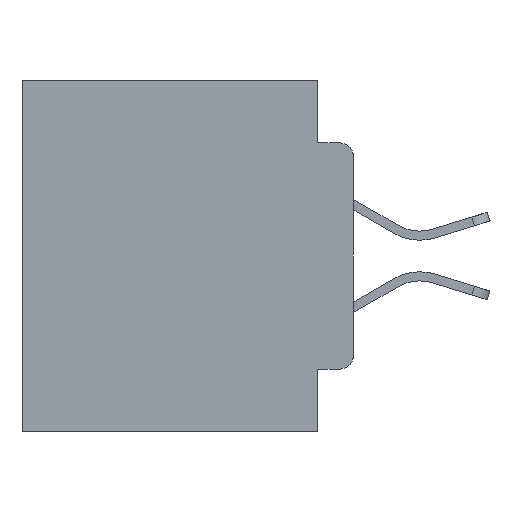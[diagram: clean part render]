
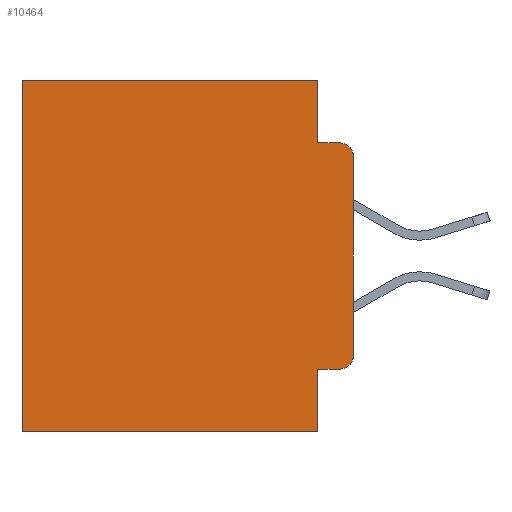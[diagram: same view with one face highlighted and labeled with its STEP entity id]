
A CAD part, left-side view. The second image highlights one B-rep face of the part: STEP entity #10464.
In plain terms, the highlighted planar face has unit normal (-1, 0, 0).
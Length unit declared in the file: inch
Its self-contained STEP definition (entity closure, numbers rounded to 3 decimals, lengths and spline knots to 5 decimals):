
#83 = EDGE_CURVE ( 'NONE', #1713, #8962, #18063, .T. ) ;
#422 = CARTESIAN_POINT ( 'NONE',  ( 0.298, 0.473, -0.5 ) ) ;
#614 = ORIENTED_EDGE ( 'NONE', *, *, #17056, .T. ) ;
#1175 = DIRECTION ( 'NONE',  ( 0., -1., 0. ) ) ;
#1609 = EDGE_CURVE ( 'NONE', #19497, #1713, #21228, .T. ) ;
#1713 = VERTEX_POINT ( 'NONE', #23904 ) ;
#1813 = ORIENTED_EDGE ( 'NONE', *, *, #6342, .T. ) ;
#1899 = ORIENTED_EDGE ( 'NONE', *, *, #4800, .F. ) ;
#2069 = VERTEX_POINT ( 'NONE', #6757 ) ;
#2101 = CARTESIAN_POINT ( 'NONE',  ( 0.298, 0.473, 0. ) ) ;
#2574 = DIRECTION ( 'NONE',  ( -1., 0., 0. ) ) ;
#2893 = VECTOR ( 'NONE', #25058, 39.37008 ) ;
#3018 = EDGE_CURVE ( 'NONE', #2069, #7826, #5050, .T. ) ;
#3116 = DIRECTION ( 'NONE',  ( 0., 1., 0. ) ) ;
#3184 = ORIENTED_EDGE ( 'NONE', *, *, #10996, .F. ) ;
#3224 = CARTESIAN_POINT ( 'NONE',  ( 0.298, 0., 0. ) ) ;
#3496 = VECTOR ( 'NONE', #6843, 39.37008 ) ;
#3650 = EDGE_LOOP ( 'NONE', ( #3685, #614, #3184, #29299, #12948, #1813, #5526, #1899, #18393, #23657 ) ) ;
#3685 = ORIENTED_EDGE ( 'NONE', *, *, #24671, .F. ) ;
#4800 = EDGE_CURVE ( 'NONE', #19497, #2069, #6781, .T. ) ;
#5050 = LINE ( 'NONE', #26342, #21846 ) ;
#5526 = ORIENTED_EDGE ( 'NONE', *, *, #3018, .F. ) ;
#5984 = EDGE_CURVE ( 'NONE', #28647, #21015, #12201, .T. ) ;
#6342 = EDGE_CURVE ( 'NONE', #21015, #7826, #27037, .T. ) ;
#6757 = CARTESIAN_POINT ( 'NONE',  ( 0.298, 0.051, -0.5 ) ) ;
#6781 = LINE ( 'NONE', #16631, #23544 ) ;
#6843 = DIRECTION ( 'NONE',  ( 0., 0., -1. ) ) ;
#7109 = DIRECTION ( 'NONE',  ( 0., 0., -1. ) ) ;
#7826 = VERTEX_POINT ( 'NONE', #422 ) ;
#8467 = CARTESIAN_POINT ( 'NONE',  ( 0.298, 0.051, -0.4115 ) ) ;
#8962 = VERTEX_POINT ( 'NONE', #25140 ) ;
#9203 = VERTEX_POINT ( 'NONE', #17669 ) ;
#9458 = EDGE_CURVE ( 'NONE', #28647, #9203, #14179, .T. ) ;
#9482 = CARTESIAN_POINT ( 'NONE',  ( 0.298, 0., -0.1085 ) ) ;
#9859 = AXIS2_PLACEMENT_3D ( 'NONE', #20017, #26807, #13266 ) ;
#10336 = CARTESIAN_POINT ( 'NONE',  ( 0.298, 0.02, -0.3915 ) ) ;
#10464 = ADVANCED_FACE ( 'NONE', ( #17997 ), #10997, .F. ) ;
#10515 = LINE ( 'NONE', #12737, #15847 ) ;
#10679 = VERTEX_POINT ( 'NONE', #9482 ) ;
#10996 = EDGE_CURVE ( 'NONE', #9203, #28455, #10515, .T. ) ;
#10997 = PLANE ( 'NONE',  #9859 ) ;
#11838 = CARTESIAN_POINT ( 'NONE',  ( 0.298, 0., 0. ) ) ;
#12201 = LINE ( 'NONE', #11838, #24267 ) ;
#12324 = CARTESIAN_POINT ( 'NONE',  ( 0.298, 0.02, -0.1085 ) ) ;
#12666 = CARTESIAN_POINT ( 'NONE',  ( 0.298, 0.051, 0. ) ) ;
#12737 = CARTESIAN_POINT ( 'NONE',  ( 0.298, 0.051, -0.0885 ) ) ;
#12948 = ORIENTED_EDGE ( 'NONE', *, *, #5984, .T. ) ;
#13078 = DIRECTION ( 'NONE',  ( 0., 0., -1. ) ) ;
#13266 = DIRECTION ( 'NONE',  ( 0., 0., -1. ) ) ;
#14179 = LINE ( 'NONE', #23072, #26190 ) ;
#14617 = DIRECTION ( 'NONE',  ( 0., 0., -1. ) ) ;
#14702 = DIRECTION ( 'NONE',  ( 0., 1., 0. ) ) ;
#15847 = VECTOR ( 'NONE', #1175, 39.37008 ) ;
#16631 = CARTESIAN_POINT ( 'NONE',  ( 0.298, 0.051, 0. ) ) ;
#17056 = EDGE_CURVE ( 'NONE', #10679, #28455, #18726, .T. ) ;
#17188 = DIRECTION ( 'NONE',  ( 0., 0., -1. ) ) ;
#17296 = CARTESIAN_POINT ( 'NONE',  ( 0.298, 0.473, 0. ) ) ;
#17669 = CARTESIAN_POINT ( 'NONE',  ( 0.298, 0.051, -0.0885 ) ) ;
#17997 = FACE_OUTER_BOUND ( 'NONE', #3650, .T. ) ;
#18063 = CIRCLE ( 'NONE', #24519, 0.02 ) ;
#18393 = ORIENTED_EDGE ( 'NONE', *, *, #1609, .T. ) ;
#18726 = CIRCLE ( 'NONE', #27370, 0.02 ) ;
#18839 = CARTESIAN_POINT ( 'NONE',  ( 0.298, 0.02, -0.0885 ) ) ;
#19280 = DIRECTION ( 'NONE',  ( 0., 0., -1. ) ) ;
#19497 = VERTEX_POINT ( 'NONE', #22235 ) ;
#20017 = CARTESIAN_POINT ( 'NONE',  ( 0.298, 0., 0. ) ) ;
#21015 = VERTEX_POINT ( 'NONE', #17296 ) ;
#21228 = LINE ( 'NONE', #8467, #2893 ) ;
#21846 = VECTOR ( 'NONE', #3116, 39.37008 ) ;
#22235 = CARTESIAN_POINT ( 'NONE',  ( 0.298, 0.051, -0.4115 ) ) ;
#23072 = CARTESIAN_POINT ( 'NONE',  ( 0.298, 0.051, 0. ) ) ;
#23544 = VECTOR ( 'NONE', #17188, 39.37008 ) ;
#23657 = ORIENTED_EDGE ( 'NONE', *, *, #83, .T. ) ;
#23904 = CARTESIAN_POINT ( 'NONE',  ( 0.298, 0.02, -0.4115 ) ) ;
#24267 = VECTOR ( 'NONE', #14702, 39.37008 ) ;
#24389 = VECTOR ( 'NONE', #19280, 39.37008 ) ;
#24519 = AXIS2_PLACEMENT_3D ( 'NONE', #10336, #2574, #13078 ) ;
#24671 = EDGE_CURVE ( 'NONE', #10679, #8962, #25117, .T. ) ;
#25058 = DIRECTION ( 'NONE',  ( 0., -1., 0. ) ) ;
#25117 = LINE ( 'NONE', #3224, #24389 ) ;
#25140 = CARTESIAN_POINT ( 'NONE',  ( 0.298, 0., -0.3915 ) ) ;
#26190 = VECTOR ( 'NONE', #7109, 39.37008 ) ;
#26342 = CARTESIAN_POINT ( 'NONE',  ( 0.298, 0., -0.5 ) ) ;
#26807 = DIRECTION ( 'NONE',  ( 1., 0., 0. ) ) ;
#27037 = LINE ( 'NONE', #2101, #3496 ) ;
#27370 = AXIS2_PLACEMENT_3D ( 'NONE', #12324, #28103, #14617 ) ;
#28103 = DIRECTION ( 'NONE',  ( -1., 0., 0. ) ) ;
#28455 = VERTEX_POINT ( 'NONE', #18839 ) ;
#28647 = VERTEX_POINT ( 'NONE', #12666 ) ;
#29299 = ORIENTED_EDGE ( 'NONE', *, *, #9458, .F. ) ;
